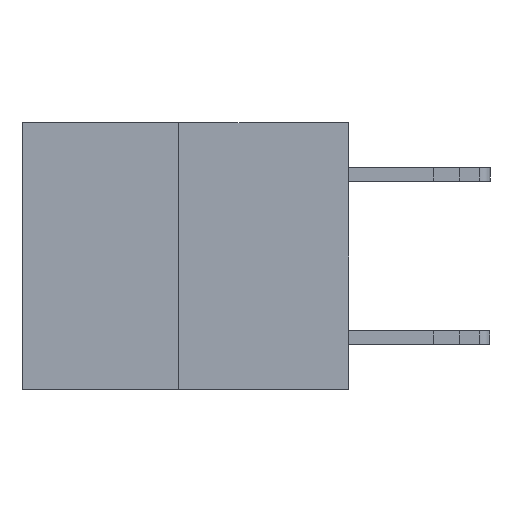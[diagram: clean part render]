
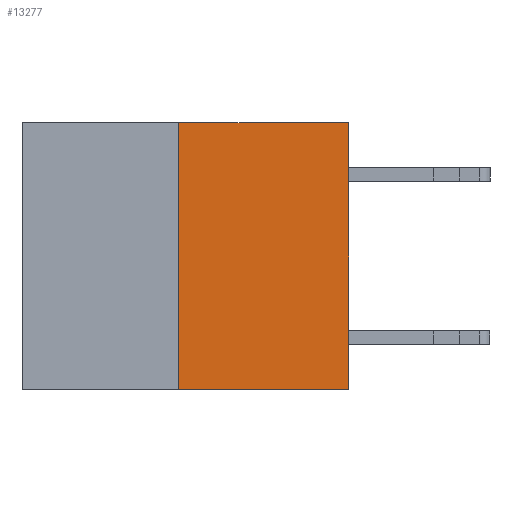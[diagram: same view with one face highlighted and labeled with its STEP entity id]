
A CAD part, left-side view. The second image highlights one B-rep face of the part: STEP entity #13277.
In plain terms, the highlighted planar face has unit normal (-1, 0, 0).
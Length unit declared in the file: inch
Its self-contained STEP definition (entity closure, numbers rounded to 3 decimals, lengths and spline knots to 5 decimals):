
#586 = ORIENTED_EDGE ( 'NONE', *, *, #2377, .T. ) ;
#861 = DIRECTION ( 'NONE',  ( 0., 0., 1. ) ) ;
#2016 = VERTEX_POINT ( 'NONE', #13042 ) ;
#2377 = EDGE_CURVE ( 'NONE', #9979, #2016, #11384, .T. ) ;
#2991 = LINE ( 'NONE', #10376, #13534 ) ;
#3057 = LINE ( 'NONE', #9671, #9734 ) ;
#3120 = DIRECTION ( 'NONE',  ( 0., 0., 1. ) ) ;
#4227 = LINE ( 'NONE', #13997, #9800 ) ;
#4376 = DIRECTION ( 'NONE',  ( 0., -1., 0. ) ) ;
#4411 = ORIENTED_EDGE ( 'NONE', *, *, #5371, .T. ) ;
#5371 = EDGE_CURVE ( 'NONE', #10498, #9979, #2991, .T. ) ;
#5461 = ORIENTED_EDGE ( 'NONE', *, *, #10469, .F. ) ;
#5990 = FACE_OUTER_BOUND ( 'NONE', #14778, .T. ) ;
#7035 = CARTESIAN_POINT ( 'NONE',  ( 0., 0., -0.49 ) ) ;
#8087 = PLANE ( 'NONE',  #8602 ) ;
#8179 = EDGE_CURVE ( 'NONE', #14639, #2016, #3057, .T. ) ;
#8326 = CARTESIAN_POINT ( 'NONE',  ( 0., 0.312, -0.49 ) ) ;
#8602 = AXIS2_PLACEMENT_3D ( 'NONE', #11693, #15222, #12735 ) ;
#9554 = VECTOR ( 'NONE', #3120, 39.37008 ) ;
#9671 = CARTESIAN_POINT ( 'NONE',  ( 0., 0.6, 0. ) ) ;
#9734 = VECTOR ( 'NONE', #14409, 39.37008 ) ;
#9800 = VECTOR ( 'NONE', #861, 39.37008 ) ;
#9979 = VERTEX_POINT ( 'NONE', #7035 ) ;
#10376 = CARTESIAN_POINT ( 'NONE',  ( 0., 0.6, -0.49 ) ) ;
#10469 = EDGE_CURVE ( 'NONE', #10498, #14639, #4227, .T. ) ;
#10498 = VERTEX_POINT ( 'NONE', #8326 ) ;
#10533 = CARTESIAN_POINT ( 'NONE',  ( 0., 0.312, 0. ) ) ;
#11384 = LINE ( 'NONE', #12720, #9554 ) ;
#11693 = CARTESIAN_POINT ( 'NONE',  ( 0., 0.6, 0. ) ) ;
#12720 = CARTESIAN_POINT ( 'NONE',  ( 0., 0., 0. ) ) ;
#12732 = ORIENTED_EDGE ( 'NONE', *, *, #8179, .F. ) ;
#12735 = DIRECTION ( 'NONE',  ( 0., 0., -1. ) ) ;
#13042 = CARTESIAN_POINT ( 'NONE',  ( 0., 0., 0. ) ) ;
#13277 = ADVANCED_FACE ( 'NONE', ( #5990 ), #8087, .F. ) ;
#13534 = VECTOR ( 'NONE', #4376, 39.37008 ) ;
#13997 = CARTESIAN_POINT ( 'NONE',  ( 0., 0.312, -0.49 ) ) ;
#14409 = DIRECTION ( 'NONE',  ( 0., -1., 0. ) ) ;
#14639 = VERTEX_POINT ( 'NONE', #10533 ) ;
#14778 = EDGE_LOOP ( 'NONE', ( #5461, #4411, #586, #12732 ) ) ;
#15222 = DIRECTION ( 'NONE',  ( 1., 0., 0. ) ) ;
